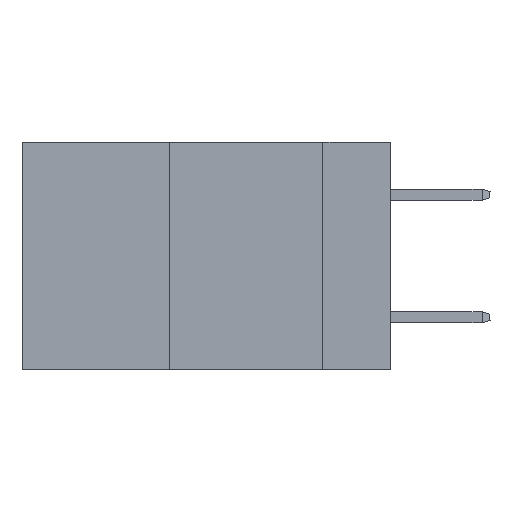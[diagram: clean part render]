
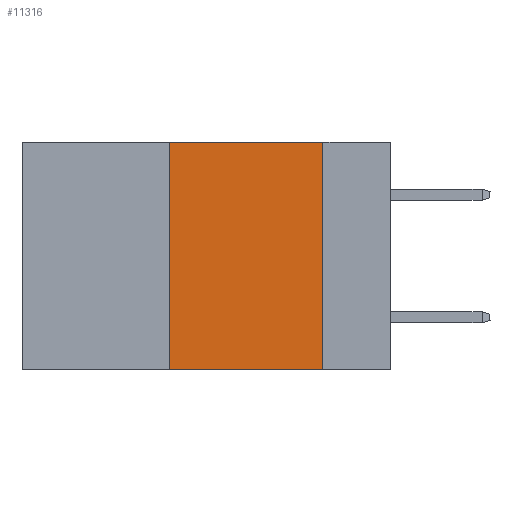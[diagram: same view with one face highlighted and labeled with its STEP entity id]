
A CAD part, left-side view. The second image highlights one B-rep face of the part: STEP entity #11316.
In plain terms, the highlighted planar face has unit normal (-1, 0, 0).
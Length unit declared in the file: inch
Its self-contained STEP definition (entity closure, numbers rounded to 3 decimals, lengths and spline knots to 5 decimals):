
#482 = CARTESIAN_POINT ( 'NONE',  ( 0., 0.6, 0. ) ) ;
#1675 = CARTESIAN_POINT ( 'NONE',  ( 0., 0.11, 0. ) ) ;
#3460 = FACE_OUTER_BOUND ( 'NONE', #29675, .T. ) ;
#3682 = PLANE ( 'NONE',  #29207 ) ;
#4448 = VECTOR ( 'NONE', #10674, 39.37008 ) ;
#6646 = VERTEX_POINT ( 'NONE', #30753 ) ;
#6876 = DIRECTION ( 'NONE',  ( 1., 0., 0. ) ) ;
#7752 = ORIENTED_EDGE ( 'NONE', *, *, #39477, .F. ) ;
#8008 = LINE ( 'NONE', #19184, #18428 ) ;
#9828 = VECTOR ( 'NONE', #26867, 39.37008 ) ;
#10674 = DIRECTION ( 'NONE',  ( 0., 0., 1. ) ) ;
#11316 = ADVANCED_FACE ( 'NONE', ( #3460 ), #3682, .F. ) ;
#11694 = VERTEX_POINT ( 'NONE', #12180 ) ;
#12180 = CARTESIAN_POINT ( 'NONE',  ( 0., 0.36, 0. ) ) ;
#13249 = ORIENTED_EDGE ( 'NONE', *, *, #34630, .F. ) ;
#13452 = EDGE_CURVE ( 'NONE', #39083, #6646, #34468, .T. ) ;
#13602 = DIRECTION ( 'NONE',  ( 0., -1., 0. ) ) ;
#16621 = VERTEX_POINT ( 'NONE', #29518 ) ;
#18289 = CARTESIAN_POINT ( 'NONE',  ( 0., 0.11, 0. ) ) ;
#18428 = VECTOR ( 'NONE', #28278, 39.37008 ) ;
#19184 = CARTESIAN_POINT ( 'NONE',  ( 0., 0.6, -0.37 ) ) ;
#23047 = LINE ( 'NONE', #28983, #31158 ) ;
#23725 = EDGE_CURVE ( 'NONE', #16621, #6646, #8008, .T. ) ;
#23905 = ORIENTED_EDGE ( 'NONE', *, *, #13452, .F. ) ;
#26867 = DIRECTION ( 'NONE',  ( 0., 0., -1. ) ) ;
#28278 = DIRECTION ( 'NONE',  ( 0., -1., 0. ) ) ;
#28681 = DIRECTION ( 'NONE',  ( 0., 0., -1. ) ) ;
#28983 = CARTESIAN_POINT ( 'NONE',  ( 0., 0.6, 0. ) ) ;
#29207 = AXIS2_PLACEMENT_3D ( 'NONE', #482, #6876, #28681 ) ;
#29373 = LINE ( 'NONE', #35329, #4448 ) ;
#29518 = CARTESIAN_POINT ( 'NONE',  ( 0., 0.36, -0.37 ) ) ;
#29675 = EDGE_LOOP ( 'NONE', ( #23905, #13249, #7752, #34409 ) ) ;
#30753 = CARTESIAN_POINT ( 'NONE',  ( 0., 0.11, -0.37 ) ) ;
#31158 = VECTOR ( 'NONE', #13602, 39.37008 ) ;
#34409 = ORIENTED_EDGE ( 'NONE', *, *, #23725, .T. ) ;
#34468 = LINE ( 'NONE', #1675, #9828 ) ;
#34630 = EDGE_CURVE ( 'NONE', #11694, #39083, #23047, .T. ) ;
#35329 = CARTESIAN_POINT ( 'NONE',  ( 0., 0.36, 0. ) ) ;
#39083 = VERTEX_POINT ( 'NONE', #18289 ) ;
#39477 = EDGE_CURVE ( 'NONE', #16621, #11694, #29373, .T. ) ;
